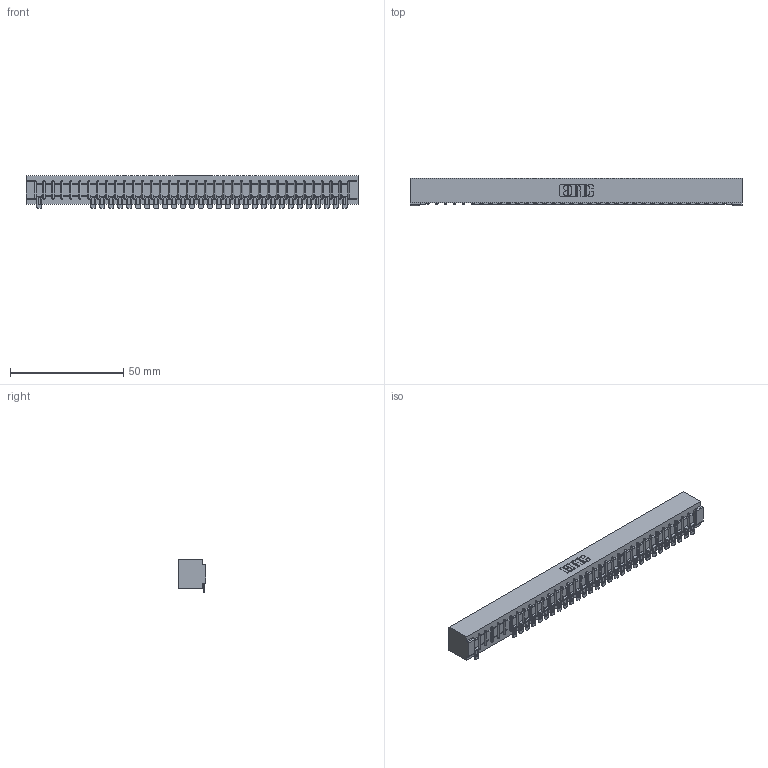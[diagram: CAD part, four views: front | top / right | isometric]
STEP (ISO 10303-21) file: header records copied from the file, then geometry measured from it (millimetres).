
FILE_DESCRIPTION (( 'STEP AP203' ), '1' );
FILE_NAME ('357-035-554-101.STEP', '2018-08-10T04:41:02', ( '' ), ( '' ), 'SwSTEP 2.0', 'SolidWorks 2016', '' );
FILE_SCHEMA (( 'CONFIG_CONTROL_DESIGN' ));
Length unit declared in the file: inch
Products named in the file (3): 307-290-002_554; 357-035-554-101; 307 Part_No Mounting Lugs
Assembly tree (31 placements, depth 2):
  357-035-554-101
    307 Part_No Mounting Lugs
    307-290-002_554  x30
Bounding box: 146.56 x 12.01 x 14.52 mm (x, y, z)
Volume: 16055.2 mm3; surface area: 19572.3 mm2
Topology: 31 solids, 31 shells, 2676 faces, 8209 edges, 5374 vertices
Faces by surface type: plane 1506, cylinder 1098, sphere 72
Entity records: 31395 total; most frequent: CARTESIAN_POINT 5317, ORIENTED_EDGE 5312, DIRECTION 5168, EDGE_CURVE 2656, LINE 2026, VECTOR 2026, VERTEX_POINT 1720, AXIS2_PLACEMENT_3D 1571
